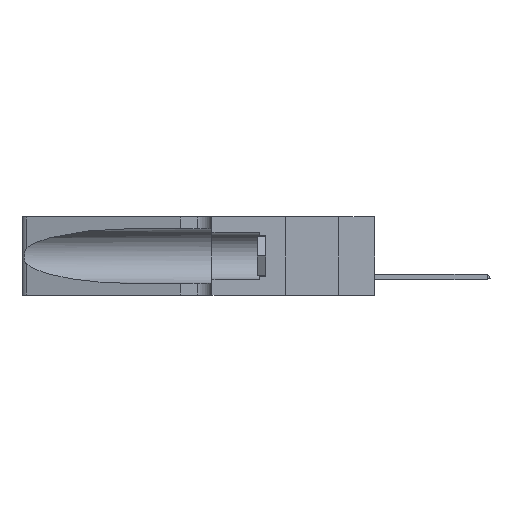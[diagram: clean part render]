
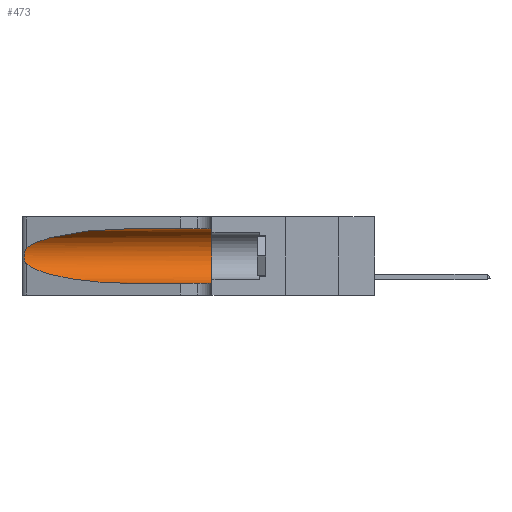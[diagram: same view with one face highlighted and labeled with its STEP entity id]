
A CAD part, left-side view. The second image highlights one B-rep face of the part: STEP entity #473.
In plain terms, the highlighted cylindrical face has radius 3.308 mm (diameter 6.617 mm), a partial arc.
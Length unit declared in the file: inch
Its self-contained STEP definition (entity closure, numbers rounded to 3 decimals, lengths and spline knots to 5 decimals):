
#473 = ADVANCED_FACE ( 'NONE', ( #22877 ), #27630, .F. ) ;
#1393 = CARTESIAN_POINT ( 'NONE',  ( 0.18966, 0.96281, 0.05475 ) ) ;
#1754 = VERTEX_POINT ( 'NONE', #15074 ) ;
#2162 = DIRECTION ( 'NONE',  ( 0., -1., 0. ) ) ;
#3029 = ORIENTED_EDGE ( 'NONE', *, *, #6699, .T. ) ;
#3843 = DIRECTION ( 'NONE',  ( 0., -1., 0. ) ) ;
#3925 = CARTESIAN_POINT ( 'NONE',  ( 0.1305, 0.35, 0.185 ) ) ;
#3998 = CARTESIAN_POINT ( 'NONE',  ( 0.25789, 1.23486, 0.15765 ) ) ;
#4428 = CARTESIAN_POINT ( 'NONE',  ( 0.25854, 1.2359, 0.20912 ) ) ;
#4484 = CARTESIAN_POINT ( 'NONE',  ( 0.1305, 0.35, 0.31525 ) ) ;
#5367 = VERTEX_POINT ( 'NONE', #23741 ) ;
#5394 = CARTESIAN_POINT ( 'NONE',  ( 0.1305, 1.61858, 0.31525 ) ) ;
#6699 = EDGE_CURVE ( 'NONE', #5367, #1754, #38222, .T. ) ;
#10106 = DIRECTION ( 'NONE',  ( 0., 0., 1. ) ) ;
#10508 = ORIENTED_EDGE ( 'NONE', *, *, #24513, .F. ) ;
#10591 = CARTESIAN_POINT ( 'NONE',  ( 0.25639, 1.23184, 0.21858 ) ) ;
#12833 = DIRECTION ( 'NONE',  ( 0., -1., 0. ) ) ;
#12968 = CARTESIAN_POINT ( 'NONE',  ( 0.25487, 1.22718, 0.14631 ) ) ;
#13373 = EDGE_CURVE ( 'NONE', #23199, #14332, #32189, .T. ) ;
#13485 = CARTESIAN_POINT ( 'NONE',  ( 0.25639, 1.23186, 0.15144 ) ) ;
#13554 = DIRECTION ( 'NONE',  ( 0., 1., 0. ) ) ;
#14332 = VERTEX_POINT ( 'NONE', #4484 ) ;
#14455 = CIRCLE ( 'NONE', #37598, 0.13025 ) ;
#14631 = CARTESIAN_POINT ( 'NONE',  ( 0.18966, 0.96281, 0.31525 ) ) ;
#15053 = EDGE_CURVE ( 'NONE', #23199, #17044, #32158, .T. ) ;
#15073 = B_SPLINE_CURVE_WITH_KNOTS ( 'NONE', 3,
 ( #34397, #37734, #10591, #22086, #4428, #17245, #38576, #37451, #22355, #22220, #3998, #13485, #25253, #28345 ),
 .UNSPECIFIED., .F., .F.,
 ( 4, 2, 2, 2, 2, 2, 4 ),
 ( 0., 0.00027, 0.00053, 0.00107, 0.0016, 0.00187, 0.00214 ),
 .UNSPECIFIED. ) ;
#15074 = CARTESIAN_POINT ( 'NONE',  ( 0.1305, 0.35, 0.05475 ) ) ;
#15222 = CARTESIAN_POINT ( 'NONE',  ( 0.25487, 1.22718, 0.22369 ) ) ;
#15829 = EDGE_LOOP ( 'NONE', ( #26167, #36403, #27236, #3029, #10508, #19942 ) ) ;
#16115 = DIRECTION ( 'NONE',  ( 0., 0., -1. ) ) ;
#17044 = VERTEX_POINT ( 'NONE', #15222 ) ;
#17245 = CARTESIAN_POINT ( 'NONE',  ( 0.26018, 1.23835, 0.19895 ) ) ;
#17646 = CARTESIAN_POINT ( 'NONE',  ( 0.25487, 1.22718, 0.14631 ) ) ;
#17686 = EDGE_CURVE ( 'NONE', #18557, #5367, #33366, .T. ) ;
#18557 = VERTEX_POINT ( 'NONE', #17646 ) ;
#19252 = VECTOR ( 'NONE', #2162, 39.37008 ) ;
#19942 = ORIENTED_EDGE ( 'NONE', *, *, #13373, .F. ) ;
#22086 = CARTESIAN_POINT ( 'NONE',  ( 0.25787, 1.23484, 0.2124 ) ) ;
#22220 = CARTESIAN_POINT ( 'NONE',  ( 0.25856, 1.23593, 0.16098 ) ) ;
#22355 = CARTESIAN_POINT ( 'NONE',  ( 0.26017, 1.23833, 0.17102 ) ) ;
#22877 = FACE_OUTER_BOUND ( 'NONE', #15829, .T. ) ;
#23199 = VERTEX_POINT ( 'NONE', #32679 ) ;
#23741 = CARTESIAN_POINT ( 'NONE',  ( 0.1305, 0.72297, 0.05475 ) ) ;
#23757 = CARTESIAN_POINT ( 'NONE',  ( 0.2373, 1.15595, 0.28018 ) ) ;
#24361 = VECTOR ( 'NONE', #12833, 39.37008 ) ;
#24513 = EDGE_CURVE ( 'NONE', #14332, #1754, #14455, .T. ) ;
#25253 = CARTESIAN_POINT ( 'NONE',  ( 0.25555, 1.22993, 0.14849 ) ) ;
#26167 = ORIENTED_EDGE ( 'NONE', *, *, #15053, .T. ) ;
#26660 = AXIS2_PLACEMENT_3D ( 'NONE', #27561, #3843, #16115 ) ;
#27236 = ORIENTED_EDGE ( 'NONE', *, *, #17686, .T. ) ;
#27561 = CARTESIAN_POINT ( 'NONE',  ( 0.1305, 1.61858, 0.185 ) ) ;
#27630 = CYLINDRICAL_SURFACE ( 'NONE', #26660, 0.13025 ) ;
#28345 = CARTESIAN_POINT ( 'NONE',  ( 0.25487, 1.22718, 0.14631 ) ) ;
#32158 =( BOUNDED_CURVE ( )  B_SPLINE_CURVE ( 3, ( #32726, #14631, #23757, #36074 ),
 .UNSPECIFIED., .F., .T. ) 
 B_SPLINE_CURVE_WITH_KNOTS ( ( 4, 4 ),
 ( 1.5708, 2.84003 ),
 .UNSPECIFIED. ) 
 CURVE ( )  GEOMETRIC_REPRESENTATION_ITEM ( )  RATIONAL_B_SPLINE_CURVE ( ( 1., 0.87, 0.87, 1. ) ) 
 REPRESENTATION_ITEM ( '' )  );
#32189 = LINE ( 'NONE', #5394, #19252 ) ;
#32679 = CARTESIAN_POINT ( 'NONE',  ( 0.1305, 0.72297, 0.31525 ) ) ;
#32726 = CARTESIAN_POINT ( 'NONE',  ( 0.1305, 0.72297, 0.31525 ) ) ;
#33366 =( BOUNDED_CURVE ( )  B_SPLINE_CURVE ( 3, ( #12968, #37914, #1393, #34446 ),
 .UNSPECIFIED., .F., .T. ) 
 B_SPLINE_CURVE_WITH_KNOTS ( ( 4, 4 ),
 ( 3.44316, 4.71239 ),
 .UNSPECIFIED. ) 
 CURVE ( )  GEOMETRIC_REPRESENTATION_ITEM ( )  RATIONAL_B_SPLINE_CURVE ( ( 1., 0.87, 0.87, 1. ) ) 
 REPRESENTATION_ITEM ( '' )  );
#34179 = CARTESIAN_POINT ( 'NONE',  ( 0.1305, 1.61858, 0.05475 ) ) ;
#34397 = CARTESIAN_POINT ( 'NONE',  ( 0.25487, 1.22718, 0.22369 ) ) ;
#34446 = CARTESIAN_POINT ( 'NONE',  ( 0.1305, 0.72297, 0.05475 ) ) ;
#36074 = CARTESIAN_POINT ( 'NONE',  ( 0.25487, 1.22718, 0.22369 ) ) ;
#36403 = ORIENTED_EDGE ( 'NONE', *, *, #38417, .T. ) ;
#37451 = CARTESIAN_POINT ( 'NONE',  ( 0.26075, 1.23896, 0.178 ) ) ;
#37598 = AXIS2_PLACEMENT_3D ( 'NONE', #3925, #13554, #10106 ) ;
#37734 = CARTESIAN_POINT ( 'NONE',  ( 0.25555, 1.22994, 0.2215 ) ) ;
#37914 = CARTESIAN_POINT ( 'NONE',  ( 0.2373, 1.15595, 0.08982 ) ) ;
#38222 = LINE ( 'NONE', #34179, #24361 ) ;
#38417 = EDGE_CURVE ( 'NONE', #17044, #18557, #15073, .T. ) ;
#38576 = CARTESIAN_POINT ( 'NONE',  ( 0.26075, 1.23896, 0.19203 ) ) ;
